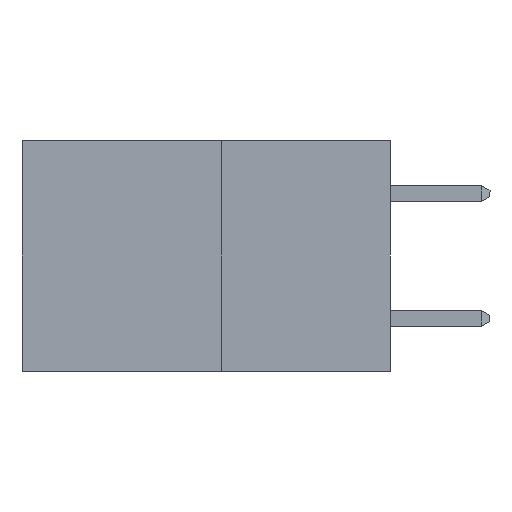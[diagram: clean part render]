
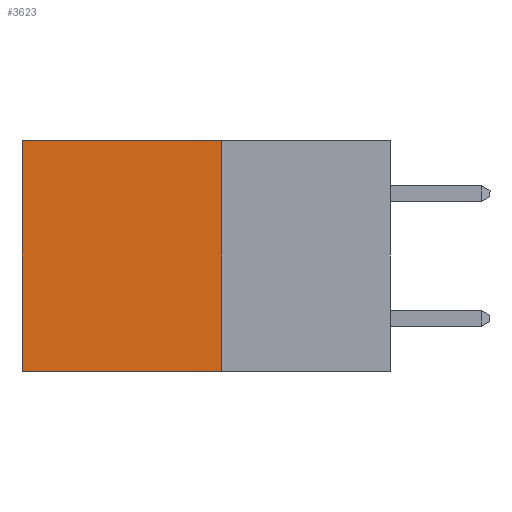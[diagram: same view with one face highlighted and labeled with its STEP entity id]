
A CAD part, left-side view. The second image highlights one B-rep face of the part: STEP entity #3623.
In plain terms, the highlighted planar face has unit normal (-1, 0, 0).
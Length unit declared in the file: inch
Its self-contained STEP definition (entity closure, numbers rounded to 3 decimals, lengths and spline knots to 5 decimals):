
#10 = DIRECTION ( 'NONE',  ( 1., 0., 0. ) ) ;
#65 = CARTESIAN_POINT ( 'NONE',  ( 0.277, 0.27, -0.37 ) ) ;
#131 = VERTEX_POINT ( 'NONE', #6868 ) ;
#215 = VERTEX_POINT ( 'NONE', #1238 ) ;
#411 = DIRECTION ( 'NONE',  ( 0., 0., -1. ) ) ;
#436 = DIRECTION ( 'NONE',  ( 0., 0., -1. ) ) ;
#564 = LINE ( 'NONE', #5418, #4040 ) ;
#565 = DIRECTION ( 'NONE',  ( 0., 1., 0. ) ) ;
#960 = EDGE_CURVE ( 'NONE', #1821, #131, #3954, .T. ) ;
#1238 = CARTESIAN_POINT ( 'NONE',  ( 0.277, 0.27, 0. ) ) ;
#1821 = VERTEX_POINT ( 'NONE', #7843 ) ;
#2303 = EDGE_CURVE ( 'NONE', #215, #1821, #564, .T. ) ;
#2419 = PLANE ( 'NONE',  #6802 ) ;
#3104 = VERTEX_POINT ( 'NONE', #4034 ) ;
#3155 = ORIENTED_EDGE ( 'NONE', *, *, #2303, .F. ) ;
#3623 = ADVANCED_FACE ( 'NONE', ( #6244 ), #2419, .F. ) ;
#3820 = LINE ( 'NONE', #4214, #7117 ) ;
#3954 = LINE ( 'NONE', #8119, #4922 ) ;
#4034 = CARTESIAN_POINT ( 'NONE',  ( 0.277, 0.59, 0. ) ) ;
#4040 = VECTOR ( 'NONE', #411, 39.37008 ) ;
#4185 = DIRECTION ( 'NONE',  ( 0., 0., -1. ) ) ;
#4214 = CARTESIAN_POINT ( 'NONE',  ( 0.277, 0.59, -0.37 ) ) ;
#4754 = ORIENTED_EDGE ( 'NONE', *, *, #960, .F. ) ;
#4906 = DIRECTION ( 'NONE',  ( 0., 1., 0. ) ) ;
#4922 = VECTOR ( 'NONE', #565, 39.37008 ) ;
#4955 = CARTESIAN_POINT ( 'NONE',  ( 0.277, 0.27, 0. ) ) ;
#5057 = EDGE_LOOP ( 'NONE', ( #7969, #4754, #3155, #5205 ) ) ;
#5205 = ORIENTED_EDGE ( 'NONE', *, *, #6719, .T. ) ;
#5418 = CARTESIAN_POINT ( 'NONE',  ( 0.277, 0.27, -0.37 ) ) ;
#6244 = FACE_OUTER_BOUND ( 'NONE', #5057, .T. ) ;
#6719 = EDGE_CURVE ( 'NONE', #215, #3104, #7026, .T. ) ;
#6802 = AXIS2_PLACEMENT_3D ( 'NONE', #65, #10, #436 ) ;
#6836 = VECTOR ( 'NONE', #4906, 39.37008 ) ;
#6868 = CARTESIAN_POINT ( 'NONE',  ( 0.277, 0.59, -0.37 ) ) ;
#6916 = EDGE_CURVE ( 'NONE', #3104, #131, #3820, .T. ) ;
#7026 = LINE ( 'NONE', #4955, #6836 ) ;
#7117 = VECTOR ( 'NONE', #4185, 39.37008 ) ;
#7843 = CARTESIAN_POINT ( 'NONE',  ( 0.277, 0.27, -0.37 ) ) ;
#7969 = ORIENTED_EDGE ( 'NONE', *, *, #6916, .T. ) ;
#8119 = CARTESIAN_POINT ( 'NONE',  ( 0.277, 0.27, -0.37 ) ) ;
